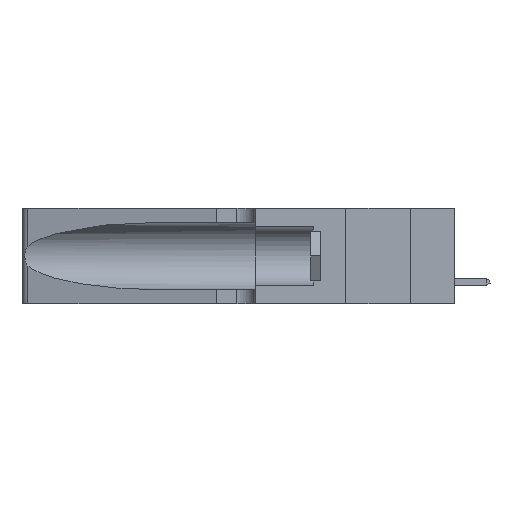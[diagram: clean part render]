
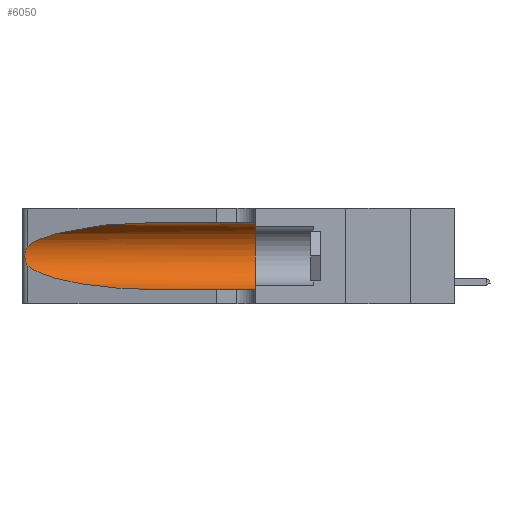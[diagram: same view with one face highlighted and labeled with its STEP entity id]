
A CAD part, left-side view. The second image highlights one B-rep face of the part: STEP entity #6050.
In plain terms, the highlighted cylindrical face has radius 3.308 mm (diameter 6.617 mm), a partial arc.
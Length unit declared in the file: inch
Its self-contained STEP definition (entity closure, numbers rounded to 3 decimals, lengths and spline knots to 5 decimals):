
#199 = ORIENTED_EDGE ( 'NONE', *, *, #3550, .T. ) ;
#558 = CARTESIAN_POINT ( 'NONE',  ( 0.1305, 0.72297, 0.31525 ) ) ;
#1047 = EDGE_CURVE ( 'NONE', #32797, #2815, #35823, .T. ) ;
#1553 = VECTOR ( 'NONE', #7781, 39.37008 ) ;
#2696 = CARTESIAN_POINT ( 'NONE',  ( 0.1305, 1.61858, 0.185 ) ) ;
#2799 = CARTESIAN_POINT ( 'NONE',  ( 0.25639, 1.23184, 0.21858 ) ) ;
#2815 = VERTEX_POINT ( 'NONE', #30274 ) ;
#3286 = CARTESIAN_POINT ( 'NONE',  ( 0.1305, 0.35, 0.05475 ) ) ;
#3550 = EDGE_CURVE ( 'NONE', #22488, #7273, #35409, .T. ) ;
#3904 = CARTESIAN_POINT ( 'NONE',  ( 0.2373, 1.15595, 0.28018 ) ) ;
#6050 = ADVANCED_FACE ( 'NONE', ( #35987 ), #45178, .F. ) ;
#6520 = DIRECTION ( 'NONE',  ( 0., -1., 0. ) ) ;
#6628 = CARTESIAN_POINT ( 'NONE',  ( 0.25854, 1.2359, 0.20912 ) ) ;
#7150 = CARTESIAN_POINT ( 'NONE',  ( 0.2373, 1.15595, 0.08982 ) ) ;
#7273 = VERTEX_POINT ( 'NONE', #3286 ) ;
#7781 = DIRECTION ( 'NONE',  ( 0., -1., 0. ) ) ;
#8517 = VERTEX_POINT ( 'NONE', #558 ) ;
#8583 = CARTESIAN_POINT ( 'NONE',  ( 0.18966, 0.96281, 0.31525 ) ) ;
#9796 = DIRECTION ( 'NONE',  ( 0., 0., 1. ) ) ;
#10313 = CARTESIAN_POINT ( 'NONE',  ( 0.26017, 1.23833, 0.17102 ) ) ;
#10621 = CARTESIAN_POINT ( 'NONE',  ( 0.26018, 1.23835, 0.19895 ) ) ;
#11832 = ORIENTED_EDGE ( 'NONE', *, *, #34086, .T. ) ;
#13752 = EDGE_CURVE ( 'NONE', #21281, #7273, #32123, .T. ) ;
#13865 = ORIENTED_EDGE ( 'NONE', *, *, #1047, .T. ) ;
#13978 = DIRECTION ( 'NONE',  ( 0., 1., 0. ) ) ;
#14619 = DIRECTION ( 'NONE',  ( 0., -1., 0. ) ) ;
#14637 = CARTESIAN_POINT ( 'NONE',  ( 0.25639, 1.23186, 0.15144 ) ) ;
#15335 = ORIENTED_EDGE ( 'NONE', *, *, #13752, .F. ) ;
#15947 = EDGE_CURVE ( 'NONE', #8517, #21281, #30808, .T. ) ;
#17510 = AXIS2_PLACEMENT_3D ( 'NONE', #43257, #13978, #9796 ) ;
#17582 = DIRECTION ( 'NONE',  ( 0., 0., -1. ) ) ;
#20267 =( BOUNDED_CURVE ( )  B_SPLINE_CURVE ( 3, ( #47078, #7150, #43674, #29268 ),
 .UNSPECIFIED., .F., .T. ) 
 B_SPLINE_CURVE_WITH_KNOTS ( ( 4, 4 ),
 ( 3.44316, 4.71239 ),
 .UNSPECIFIED. ) 
 CURVE ( )  GEOMETRIC_REPRESENTATION_ITEM ( )  RATIONAL_B_SPLINE_CURVE ( ( 1., 0.87, 0.87, 1. ) ) 
 REPRESENTATION_ITEM ( '' )  );
#21042 = VECTOR ( 'NONE', #14619, 39.37008 ) ;
#21106 = CARTESIAN_POINT ( 'NONE',  ( 0.1305, 1.61858, 0.31525 ) ) ;
#21281 = VERTEX_POINT ( 'NONE', #46667 ) ;
#22488 = VERTEX_POINT ( 'NONE', #31384 ) ;
#23334 = ORIENTED_EDGE ( 'NONE', *, *, #25804, .T. ) ;
#24914 = CARTESIAN_POINT ( 'NONE',  ( 0.25555, 1.22994, 0.2215 ) ) ;
#25225 = CARTESIAN_POINT ( 'NONE',  ( 0.25789, 1.23486, 0.15765 ) ) ;
#25701 = CARTESIAN_POINT ( 'NONE',  ( 0.25487, 1.22718, 0.14631 ) ) ;
#25804 = EDGE_CURVE ( 'NONE', #8517, #32797, #44936, .T. ) ;
#26852 = CARTESIAN_POINT ( 'NONE',  ( 0.1305, 0.72297, 0.31525 ) ) ;
#28585 = CARTESIAN_POINT ( 'NONE',  ( 0.25787, 1.23484, 0.2124 ) ) ;
#28906 = CARTESIAN_POINT ( 'NONE',  ( 0.25856, 1.23593, 0.16098 ) ) ;
#29214 = CARTESIAN_POINT ( 'NONE',  ( 0.25555, 1.22993, 0.14849 ) ) ;
#29268 = CARTESIAN_POINT ( 'NONE',  ( 0.1305, 0.72297, 0.05475 ) ) ;
#30274 = CARTESIAN_POINT ( 'NONE',  ( 0.25487, 1.22718, 0.14631 ) ) ;
#30546 = AXIS2_PLACEMENT_3D ( 'NONE', #2696, #6520, #17582 ) ;
#30808 = LINE ( 'NONE', #21106, #1553 ) ;
#31384 = CARTESIAN_POINT ( 'NONE',  ( 0.1305, 0.72297, 0.05475 ) ) ;
#32123 = CIRCLE ( 'NONE', #17510, 0.13025 ) ;
#32297 = CARTESIAN_POINT ( 'NONE',  ( 0.26075, 1.23896, 0.19203 ) ) ;
#32797 = VERTEX_POINT ( 'NONE', #44276 ) ;
#32917 = CARTESIAN_POINT ( 'NONE',  ( 0.25487, 1.22718, 0.22369 ) ) ;
#34086 = EDGE_CURVE ( 'NONE', #2815, #22488, #20267, .T. ) ;
#35409 = LINE ( 'NONE', #43609, #21042 ) ;
#35823 = B_SPLINE_CURVE_WITH_KNOTS ( 'NONE', 3,
 ( #46874, #24914, #2799, #28585, #6628, #10621, #32297, #47173, #10313, #28906, #25225, #14637, #29214, #25701 ),
 .UNSPECIFIED., .F., .F.,
 ( 4, 2, 2, 2, 2, 2, 4 ),
 ( 0., 0.00027, 0.00053, 0.00107, 0.0016, 0.00187, 0.00214 ),
 .UNSPECIFIED. ) ;
#35987 = FACE_OUTER_BOUND ( 'NONE', #36040, .T. ) ;
#36040 = EDGE_LOOP ( 'NONE', ( #23334, #13865, #11832, #199, #15335, #38057 ) ) ;
#38057 = ORIENTED_EDGE ( 'NONE', *, *, #15947, .F. ) ;
#43257 = CARTESIAN_POINT ( 'NONE',  ( 0.1305, 0.35, 0.185 ) ) ;
#43609 = CARTESIAN_POINT ( 'NONE',  ( 0.1305, 1.61858, 0.05475 ) ) ;
#43674 = CARTESIAN_POINT ( 'NONE',  ( 0.18966, 0.96281, 0.05475 ) ) ;
#44276 = CARTESIAN_POINT ( 'NONE',  ( 0.25487, 1.22718, 0.22369 ) ) ;
#44936 =( BOUNDED_CURVE ( )  B_SPLINE_CURVE ( 3, ( #26852, #8583, #3904, #32917 ),
 .UNSPECIFIED., .F., .T. ) 
 B_SPLINE_CURVE_WITH_KNOTS ( ( 4, 4 ),
 ( 1.5708, 2.84003 ),
 .UNSPECIFIED. ) 
 CURVE ( )  GEOMETRIC_REPRESENTATION_ITEM ( )  RATIONAL_B_SPLINE_CURVE ( ( 1., 0.87, 0.87, 1. ) ) 
 REPRESENTATION_ITEM ( '' )  );
#45178 = CYLINDRICAL_SURFACE ( 'NONE', #30546, 0.13025 ) ;
#46667 = CARTESIAN_POINT ( 'NONE',  ( 0.1305, 0.35, 0.31525 ) ) ;
#46874 = CARTESIAN_POINT ( 'NONE',  ( 0.25487, 1.22718, 0.22369 ) ) ;
#47078 = CARTESIAN_POINT ( 'NONE',  ( 0.25487, 1.22718, 0.14631 ) ) ;
#47173 = CARTESIAN_POINT ( 'NONE',  ( 0.26075, 1.23896, 0.178 ) ) ;
